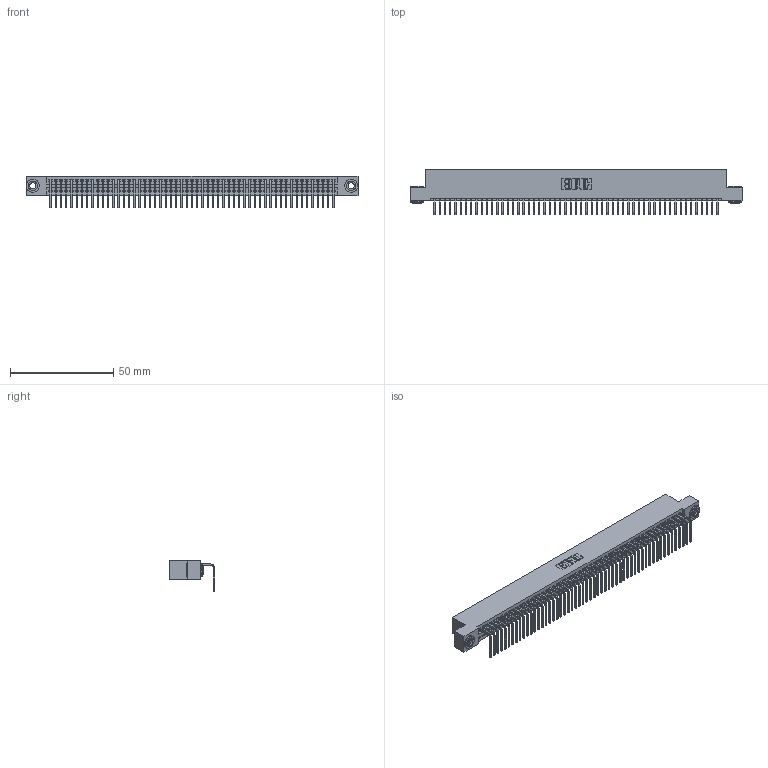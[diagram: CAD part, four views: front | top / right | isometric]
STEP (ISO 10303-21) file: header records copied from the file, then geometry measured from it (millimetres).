
FILE_DESCRIPTION (( 'STEP AP203' ), '1' );
FILE_NAME ('395-055-558-103.STEP', '2019-10-11T14:52:06', ( '' ), ( '' ), 'SwSTEP 2.0', 'SolidWorks 2016', '' );
FILE_SCHEMA (( 'CONFIG_CONTROL_DESIGN' ));
Length unit declared in the file: inch
Products named in the file (4): 345 Part_Flush Mounting Lugs - 0.156 Dia-TH; 345-292-001_558 Tail - 2; 345-250-002_345-250-002-102; 395-055-558-103
Assembly tree (58 placements, depth 2):
  395-055-558-103
    345 Part_Flush Mounting Lugs - 0.156 Dia-TH
    345-292-001_558 Tail - 2  x55
    345-250-002_345-250-002-102  x2
Bounding box: 160.91 x 21.83 x 15.37 mm (x, y, z)
Volume: 15592.4 mm3; surface area: 22188.9 mm2
Topology: 58 solids, 58 shells, 3464 faces, 10427 edges, 6874 vertices
Faces by surface type: plane 2400, cylinder 1056, cone 8
Entity records: 40378 total; most frequent: CARTESIAN_POINT 6972, ORIENTED_EDGE 6954, DIRECTION 6101, EDGE_CURVE 3477, LINE 3101, VECTOR 3101, VERTEX_POINT 2314, AXIS2_PLACEMENT_3D 1500
